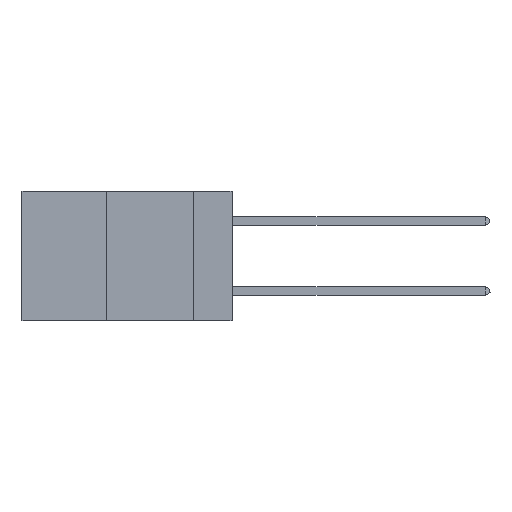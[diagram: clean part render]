
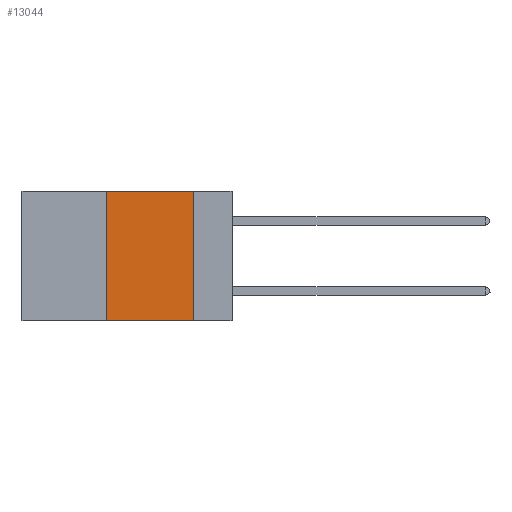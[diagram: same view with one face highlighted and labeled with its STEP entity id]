
A CAD part, left-side view. The second image highlights one B-rep face of the part: STEP entity #13044.
In plain terms, the highlighted planar face has unit normal (-1, 0, 0).
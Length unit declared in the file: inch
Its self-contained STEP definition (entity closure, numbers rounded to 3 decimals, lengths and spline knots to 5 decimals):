
#36 = VECTOR ( 'NONE', #8245, 39.37008 ) ;
#44 = VERTEX_POINT ( 'NONE', #1376 ) ;
#1151 = ORIENTED_EDGE ( 'NONE', *, *, #2306, .F. ) ;
#1376 = CARTESIAN_POINT ( 'NONE',  ( 0., 0.11, 0. ) ) ;
#1828 = FACE_OUTER_BOUND ( 'NONE', #3036, .T. ) ;
#1907 = CARTESIAN_POINT ( 'NONE',  ( 0., 0.36, 0. ) ) ;
#2002 = CARTESIAN_POINT ( 'NONE',  ( 0., 0.11, 0. ) ) ;
#2177 = VECTOR ( 'NONE', #5145, 39.37008 ) ;
#2306 = EDGE_CURVE ( 'NONE', #44, #8660, #13150, .T. ) ;
#2616 = EDGE_CURVE ( 'NONE', #8418, #8660, #8093, .T. ) ;
#3036 = EDGE_LOOP ( 'NONE', ( #1151, #11095, #13060, #6775 ) ) ;
#3592 = CARTESIAN_POINT ( 'NONE',  ( 0., 0.36, 0. ) ) ;
#4812 = LINE ( 'NONE', #9256, #2177 ) ;
#5145 = DIRECTION ( 'NONE',  ( 0., -1., 0. ) ) ;
#5410 = CARTESIAN_POINT ( 'NONE',  ( 0., 0.11, -0.37 ) ) ;
#6674 = DIRECTION ( 'NONE',  ( 0., -1., 0. ) ) ;
#6775 = ORIENTED_EDGE ( 'NONE', *, *, #2616, .T. ) ;
#7473 = DIRECTION ( 'NONE',  ( 1., 0., 0. ) ) ;
#8093 = LINE ( 'NONE', #12855, #10034 ) ;
#8245 = DIRECTION ( 'NONE',  ( 0., 0., 1. ) ) ;
#8296 = CARTESIAN_POINT ( 'NONE',  ( 0., 0.36, -0.37 ) ) ;
#8418 = VERTEX_POINT ( 'NONE', #8296 ) ;
#8465 = PLANE ( 'NONE',  #8724 ) ;
#8594 = CARTESIAN_POINT ( 'NONE',  ( 0., 0.6, 0. ) ) ;
#8660 = VERTEX_POINT ( 'NONE', #5410 ) ;
#8724 = AXIS2_PLACEMENT_3D ( 'NONE', #8594, #7473, #12753 ) ;
#9256 = CARTESIAN_POINT ( 'NONE',  ( 0., 0.6, 0. ) ) ;
#10034 = VECTOR ( 'NONE', #6674, 39.37008 ) ;
#10383 = VECTOR ( 'NONE', #12310, 39.37008 ) ;
#11095 = ORIENTED_EDGE ( 'NONE', *, *, #12320, .F. ) ;
#11906 = VERTEX_POINT ( 'NONE', #3592 ) ;
#12262 = EDGE_CURVE ( 'NONE', #8418, #11906, #12920, .T. ) ;
#12310 = DIRECTION ( 'NONE',  ( 0., 0., -1. ) ) ;
#12320 = EDGE_CURVE ( 'NONE', #11906, #44, #4812, .T. ) ;
#12753 = DIRECTION ( 'NONE',  ( 0., 0., -1. ) ) ;
#12855 = CARTESIAN_POINT ( 'NONE',  ( 0., 0.6, -0.37 ) ) ;
#12920 = LINE ( 'NONE', #1907, #36 ) ;
#13044 = ADVANCED_FACE ( 'NONE', ( #1828 ), #8465, .F. ) ;
#13060 = ORIENTED_EDGE ( 'NONE', *, *, #12262, .F. ) ;
#13150 = LINE ( 'NONE', #2002, #10383 ) ;
